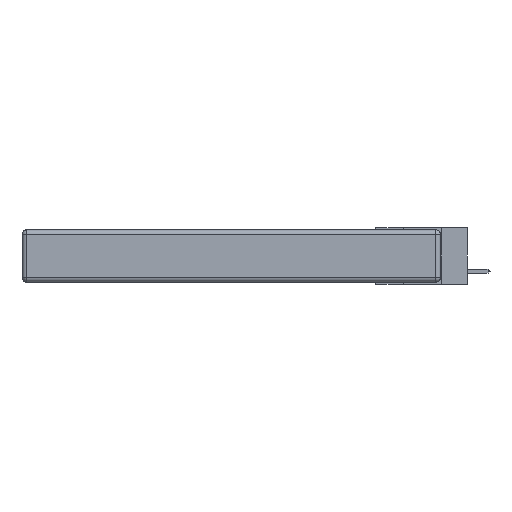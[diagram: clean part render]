
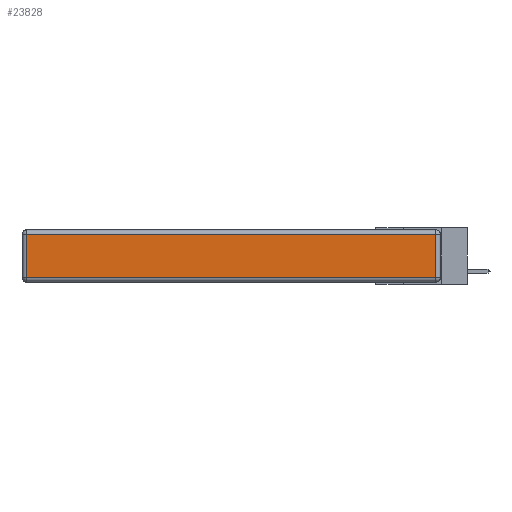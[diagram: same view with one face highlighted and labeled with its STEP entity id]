
A CAD part, left-side view. The second image highlights one B-rep face of the part: STEP entity #23828.
In plain terms, the highlighted planar face has unit normal (-1, 0, 0).
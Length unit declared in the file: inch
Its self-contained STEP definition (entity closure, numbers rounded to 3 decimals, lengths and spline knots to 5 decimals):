
#175 = ORIENTED_EDGE ( 'NONE', *, *, #23580, .T. ) ;
#317 = DIRECTION ( 'NONE',  ( -1., 0., 0. ) ) ;
#1089 = CARTESIAN_POINT ( 'NONE',  ( 0., 2.72, -0.313 ) ) ;
#1717 = CARTESIAN_POINT ( 'NONE',  ( 0., 2.75, -0.03 ) ) ;
#2580 = DIRECTION ( 'NONE',  ( 0., 0., 1. ) ) ;
#4655 = DIRECTION ( 'NONE',  ( 0., 0., 1. ) ) ;
#7354 = EDGE_LOOP ( 'NONE', ( #9236, #25689, #175, #12881 ) ) ;
#7376 = LINE ( 'NONE', #17272, #26441 ) ;
#7700 = VECTOR ( 'NONE', #4655, 39.37008 ) ;
#9185 = LINE ( 'NONE', #30329, #7700 ) ;
#9236 = ORIENTED_EDGE ( 'NONE', *, *, #9517, .T. ) ;
#9500 = CARTESIAN_POINT ( 'NONE',  ( 0., 2.72, -0.03 ) ) ;
#9517 = EDGE_CURVE ( 'NONE', #24951, #12901, #7376, .T. ) ;
#10052 = CARTESIAN_POINT ( 'NONE',  ( 0., 2.72, -0.343 ) ) ;
#11800 = VERTEX_POINT ( 'NONE', #9500 ) ;
#11803 = PLANE ( 'NONE',  #22596 ) ;
#12564 = LINE ( 'NONE', #1717, #26852 ) ;
#12881 = ORIENTED_EDGE ( 'NONE', *, *, #23285, .T. ) ;
#12901 = VERTEX_POINT ( 'NONE', #18482 ) ;
#14727 = LINE ( 'NONE', #10052, #18803 ) ;
#14900 = DIRECTION ( 'NONE',  ( 0., 0., -1. ) ) ;
#15002 = CARTESIAN_POINT ( 'NONE',  ( 0., 0.03, -0.03 ) ) ;
#17272 = CARTESIAN_POINT ( 'NONE',  ( 0., 0., -0.313 ) ) ;
#17563 = VERTEX_POINT ( 'NONE', #15002 ) ;
#18128 = DIRECTION ( 'NONE',  ( 0., 1., 0. ) ) ;
#18419 = EDGE_CURVE ( 'NONE', #12901, #17563, #9185, .T. ) ;
#18482 = CARTESIAN_POINT ( 'NONE',  ( 0., 0.03, -0.313 ) ) ;
#18803 = VECTOR ( 'NONE', #14900, 39.37008 ) ;
#19721 = DIRECTION ( 'NONE',  ( 0., -1., 0. ) ) ;
#22596 = AXIS2_PLACEMENT_3D ( 'NONE', #27948, #317, #2580 ) ;
#23285 = EDGE_CURVE ( 'NONE', #11800, #24951, #14727, .T. ) ;
#23580 = EDGE_CURVE ( 'NONE', #17563, #11800, #12564, .T. ) ;
#23828 = ADVANCED_FACE ( 'NONE', ( #28383 ), #11803, .T. ) ;
#24951 = VERTEX_POINT ( 'NONE', #1089 ) ;
#25689 = ORIENTED_EDGE ( 'NONE', *, *, #18419, .T. ) ;
#26441 = VECTOR ( 'NONE', #19721, 39.37008 ) ;
#26852 = VECTOR ( 'NONE', #18128, 39.37008 ) ;
#27948 = CARTESIAN_POINT ( 'NONE',  ( 0., 0., -0.343 ) ) ;
#28383 = FACE_OUTER_BOUND ( 'NONE', #7354, .T. ) ;
#30329 = CARTESIAN_POINT ( 'NONE',  ( 0., 0.03, -0.343 ) ) ;
